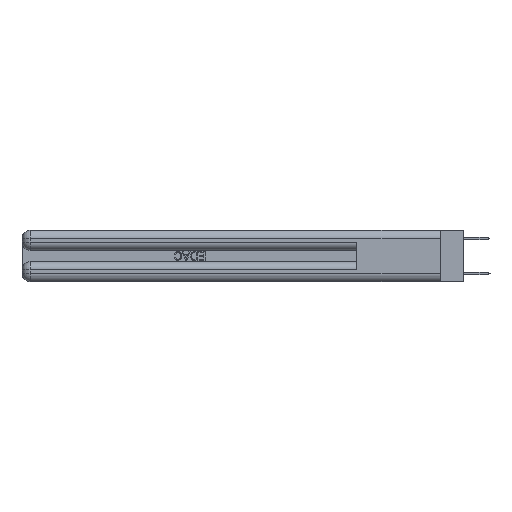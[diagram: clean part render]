
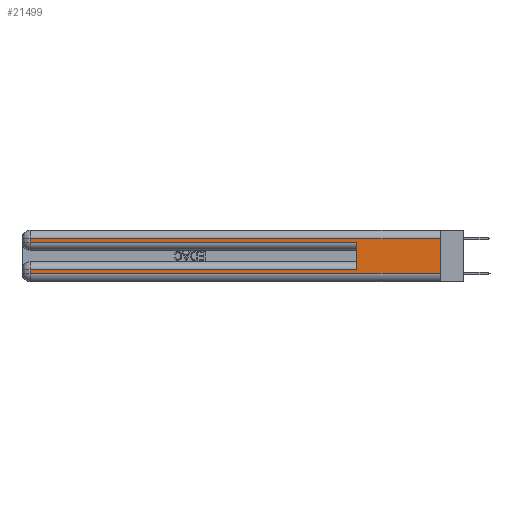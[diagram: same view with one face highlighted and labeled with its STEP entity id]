
A CAD part, left-side view. The second image highlights one B-rep face of the part: STEP entity #21499.
In plain terms, the highlighted planar face has unit normal (-1, 0, 0).
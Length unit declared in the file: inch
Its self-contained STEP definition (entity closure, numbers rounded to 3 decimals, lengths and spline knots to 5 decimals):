
#1645 = CARTESIAN_POINT ( 'NONE',  ( 0., 0., 0.285 ) ) ;
#1819 = ORIENTED_EDGE ( 'NONE', *, *, #16101, .T. ) ;
#2032 = DIRECTION ( 'NONE',  ( 0., 1., 0. ) ) ;
#2121 = LINE ( 'NONE', #1645, #28614 ) ;
#2197 = LINE ( 'NONE', #4653, #21769 ) ;
#2679 = VERTEX_POINT ( 'NONE', #31769 ) ;
#2744 = CARTESIAN_POINT ( 'NONE',  ( 0., 2.94, 0.37 ) ) ;
#2885 = CARTESIAN_POINT ( 'NONE',  ( 0., 0., 0.31 ) ) ;
#2998 = DIRECTION ( 'NONE',  ( 0., 1., 0. ) ) ;
#3124 = DIRECTION ( 'NONE',  ( 1., 0., 0. ) ) ;
#4509 = CARTESIAN_POINT ( 'NONE',  ( 0., 2.94, 0.37 ) ) ;
#4653 = CARTESIAN_POINT ( 'NONE',  ( 0., 0., 0.37 ) ) ;
#5159 = EDGE_CURVE ( 'NONE', #20680, #2679, #2197, .T. ) ;
#5523 = LINE ( 'NONE', #31901, #26719 ) ;
#5741 = DIRECTION ( 'NONE',  ( 0., 0., -1. ) ) ;
#5941 = CARTESIAN_POINT ( 'NONE',  ( 0., 2.94, 0.285 ) ) ;
#7399 = CARTESIAN_POINT ( 'NONE',  ( 0., 2.94, 0.06 ) ) ;
#7677 = VERTEX_POINT ( 'NONE', #16603 ) ;
#8044 = EDGE_CURVE ( 'NONE', #22501, #2679, #5523, .T. ) ;
#8120 = EDGE_CURVE ( 'NONE', #8496, #22501, #12870, .T. ) ;
#8496 = VERTEX_POINT ( 'NONE', #30456 ) ;
#8550 = CARTESIAN_POINT ( 'NONE',  ( 0., 0., 0.31 ) ) ;
#10676 = VERTEX_POINT ( 'NONE', #30243 ) ;
#12074 = DIRECTION ( 'NONE',  ( 0., -1., 0. ) ) ;
#12132 = CARTESIAN_POINT ( 'NONE',  ( 0., 0., 0.085 ) ) ;
#12341 = ORIENTED_EDGE ( 'NONE', *, *, #5159, .F. ) ;
#12703 = DIRECTION ( 'NONE',  ( 0., 0., -1. ) ) ;
#12870 = LINE ( 'NONE', #2744, #27477 ) ;
#12904 = ORIENTED_EDGE ( 'NONE', *, *, #8044, .T. ) ;
#13154 = LINE ( 'NONE', #15943, #26803 ) ;
#14324 = VECTOR ( 'NONE', #24446, 39.37008 ) ;
#14804 = VERTEX_POINT ( 'NONE', #31538 ) ;
#15482 = DIRECTION ( 'NONE',  ( 0., -1., 0. ) ) ;
#15543 = FACE_OUTER_BOUND ( 'NONE', #23378, .T. ) ;
#15943 = CARTESIAN_POINT ( 'NONE',  ( 0., 0.6, 0.145 ) ) ;
#16101 = EDGE_CURVE ( 'NONE', #20680, #7677, #23417, .T. ) ;
#16603 = CARTESIAN_POINT ( 'NONE',  ( 0., 2.94, 0.31 ) ) ;
#16608 = LINE ( 'NONE', #4509, #14324 ) ;
#18117 = EDGE_CURVE ( 'NONE', #10676, #14804, #13154, .T. ) ;
#18476 = CARTESIAN_POINT ( 'NONE',  ( 0., 0., 0.37 ) ) ;
#19549 = EDGE_CURVE ( 'NONE', #7677, #19881, #16608, .T. ) ;
#19881 = VERTEX_POINT ( 'NONE', #5941 ) ;
#20680 = VERTEX_POINT ( 'NONE', #2885 ) ;
#21499 = ADVANCED_FACE ( 'NONE', ( #15543 ), #25509, .F. ) ;
#21769 = VECTOR ( 'NONE', #22591, 39.37008 ) ;
#22461 = EDGE_CURVE ( 'NONE', #10676, #8496, #29162, .T. ) ;
#22501 = VERTEX_POINT ( 'NONE', #7399 ) ;
#22591 = DIRECTION ( 'NONE',  ( 0., 0., -1. ) ) ;
#23378 = EDGE_LOOP ( 'NONE', ( #12341, #1819, #29427, #24168, #25794, #25313, #26116, #12904 ) ) ;
#23417 = LINE ( 'NONE', #8550, #31160 ) ;
#23700 = AXIS2_PLACEMENT_3D ( 'NONE', #18476, #3124, #5741 ) ;
#24168 = ORIENTED_EDGE ( 'NONE', *, *, #29339, .T. ) ;
#24446 = DIRECTION ( 'NONE',  ( 0., 0., -1. ) ) ;
#25313 = ORIENTED_EDGE ( 'NONE', *, *, #22461, .T. ) ;
#25509 = PLANE ( 'NONE',  #23700 ) ;
#25794 = ORIENTED_EDGE ( 'NONE', *, *, #18117, .F. ) ;
#26116 = ORIENTED_EDGE ( 'NONE', *, *, #8120, .T. ) ;
#26719 = VECTOR ( 'NONE', #15482, 39.37008 ) ;
#26803 = VECTOR ( 'NONE', #28539, 39.37008 ) ;
#27477 = VECTOR ( 'NONE', #12703, 39.37008 ) ;
#28539 = DIRECTION ( 'NONE',  ( 0., 0., 1. ) ) ;
#28614 = VECTOR ( 'NONE', #12074, 39.37008 ) ;
#29003 = VECTOR ( 'NONE', #2032, 39.37008 ) ;
#29162 = LINE ( 'NONE', #12132, #29003 ) ;
#29339 = EDGE_CURVE ( 'NONE', #19881, #14804, #2121, .T. ) ;
#29427 = ORIENTED_EDGE ( 'NONE', *, *, #19549, .T. ) ;
#30243 = CARTESIAN_POINT ( 'NONE',  ( 0., 0.6, 0.085 ) ) ;
#30456 = CARTESIAN_POINT ( 'NONE',  ( 0., 2.94, 0.085 ) ) ;
#31160 = VECTOR ( 'NONE', #2998, 39.37008 ) ;
#31538 = CARTESIAN_POINT ( 'NONE',  ( 0., 0.6, 0.285 ) ) ;
#31769 = CARTESIAN_POINT ( 'NONE',  ( 0., 0., 0.06 ) ) ;
#31901 = CARTESIAN_POINT ( 'NONE',  ( 0., 0., 0.06 ) ) ;
